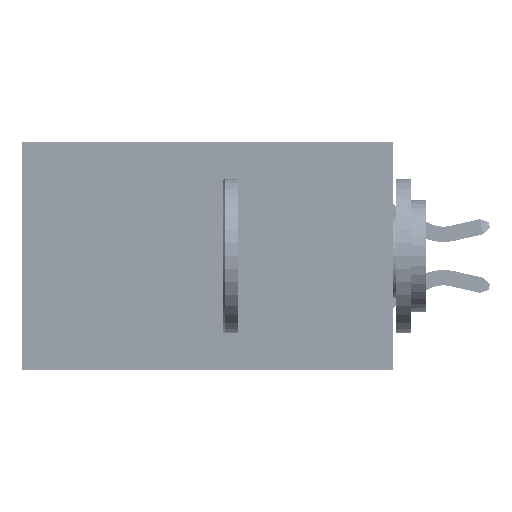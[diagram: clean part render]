
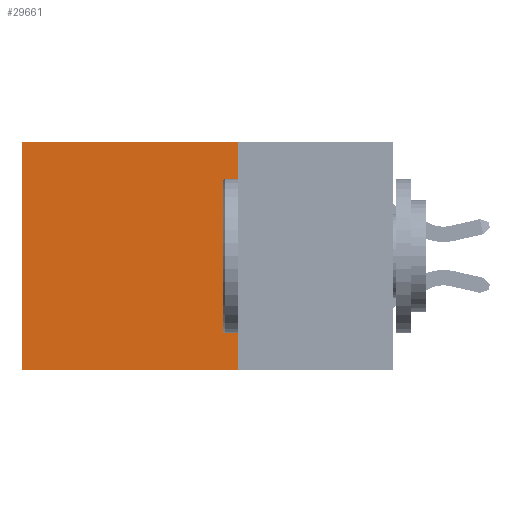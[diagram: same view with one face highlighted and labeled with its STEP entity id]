
A CAD part, left-side view. The second image highlights one B-rep face of the part: STEP entity #29661.
In plain terms, the highlighted planar face has unit normal (-1, 0, 0).
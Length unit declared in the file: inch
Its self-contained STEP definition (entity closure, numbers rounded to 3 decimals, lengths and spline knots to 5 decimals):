
#1963 = CARTESIAN_POINT ( 'NONE',  ( 0.2875, 0.25, 0. ) ) ;
#2126 = DIRECTION ( 'NONE',  ( 0., 0., -1. ) ) ;
#3808 = DIRECTION ( 'NONE',  ( 0., 0., -1. ) ) ;
#5148 = DIRECTION ( 'NONE',  ( 0., 1., 0. ) ) ;
#9195 = VECTOR ( 'NONE', #5148, 39.37008 ) ;
#9675 = CARTESIAN_POINT ( 'NONE',  ( 0.2875, 0.6, -0.37 ) ) ;
#11286 = EDGE_LOOP ( 'NONE', ( #41210, #23181, #24862, #46065 ) ) ;
#11506 = CARTESIAN_POINT ( 'NONE',  ( 0.2875, 0.25, 0. ) ) ;
#13519 = DIRECTION ( 'NONE',  ( 1., 0., 0. ) ) ;
#17458 = LINE ( 'NONE', #11506, #26362 ) ;
#17599 = LINE ( 'NONE', #47389, #9195 ) ;
#17989 = EDGE_CURVE ( 'NONE', #36126, #34536, #17599, .T. ) ;
#19355 = DIRECTION ( 'NONE',  ( 0., 1., 0. ) ) ;
#22611 = VECTOR ( 'NONE', #19355, 39.37008 ) ;
#23181 = ORIENTED_EDGE ( 'NONE', *, *, #40172, .F. ) ;
#23401 = CARTESIAN_POINT ( 'NONE',  ( 0.2875, 0.25, -0.37 ) ) ;
#24556 = PLANE ( 'NONE',  #30797 ) ;
#24862 = ORIENTED_EDGE ( 'NONE', *, *, #45674, .F. ) ;
#24926 = VECTOR ( 'NONE', #32980, 39.37008 ) ;
#26362 = VECTOR ( 'NONE', #3808, 39.37008 ) ;
#29661 = ADVANCED_FACE ( 'NONE', ( #38192 ), #24556, .F. ) ;
#30797 = AXIS2_PLACEMENT_3D ( 'NONE', #1963, #13519, #2126 ) ;
#32768 = LINE ( 'NONE', #37884, #22611 ) ;
#32980 = DIRECTION ( 'NONE',  ( 0., 0., -1. ) ) ;
#33820 = LINE ( 'NONE', #40986, #24926 ) ;
#33901 = VERTEX_POINT ( 'NONE', #23401 ) ;
#34536 = VERTEX_POINT ( 'NONE', #49290 ) ;
#36126 = VERTEX_POINT ( 'NONE', #46210 ) ;
#36244 = VERTEX_POINT ( 'NONE', #9675 ) ;
#37884 = CARTESIAN_POINT ( 'NONE',  ( 0.2875, 0.25, -0.37 ) ) ;
#38192 = FACE_OUTER_BOUND ( 'NONE', #11286, .T. ) ;
#40172 = EDGE_CURVE ( 'NONE', #33901, #36244, #32768, .T. ) ;
#40986 = CARTESIAN_POINT ( 'NONE',  ( 0.2875, 0.6, 0. ) ) ;
#41100 = EDGE_CURVE ( 'NONE', #34536, #36244, #33820, .T. ) ;
#41210 = ORIENTED_EDGE ( 'NONE', *, *, #41100, .T. ) ;
#45674 = EDGE_CURVE ( 'NONE', #36126, #33901, #17458, .T. ) ;
#46065 = ORIENTED_EDGE ( 'NONE', *, *, #17989, .T. ) ;
#46210 = CARTESIAN_POINT ( 'NONE',  ( 0.2875, 0.25, 0. ) ) ;
#47389 = CARTESIAN_POINT ( 'NONE',  ( 0.2875, 0.25, 0. ) ) ;
#49290 = CARTESIAN_POINT ( 'NONE',  ( 0.2875, 0.6, 0. ) ) ;
